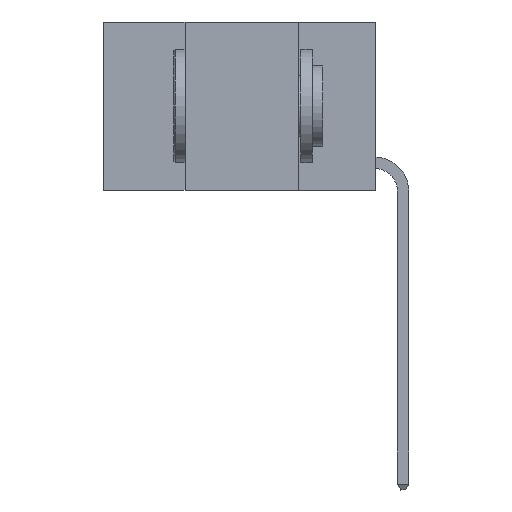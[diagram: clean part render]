
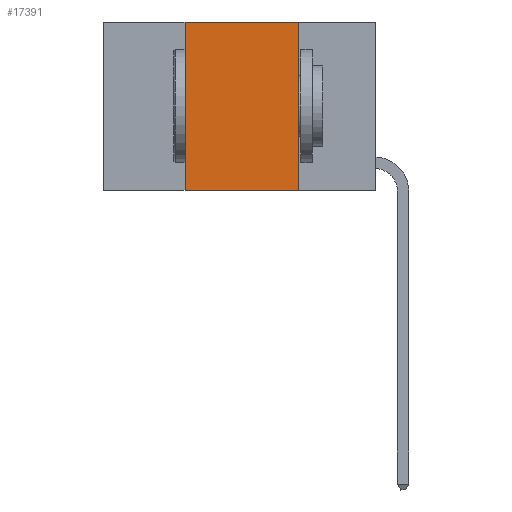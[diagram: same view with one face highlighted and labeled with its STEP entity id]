
A CAD part, left-side view. The second image highlights one B-rep face of the part: STEP entity #17391.
In plain terms, the highlighted planar face has unit normal (-1, 0, 0).
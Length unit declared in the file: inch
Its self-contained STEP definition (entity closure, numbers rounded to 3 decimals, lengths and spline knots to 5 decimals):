
#11 = CARTESIAN_POINT ( 'NONE',  ( 0., 0.17, 0. ) ) ;
#609 = EDGE_CURVE ( 'NONE', #15413, #7336, #24005, .T. ) ;
#3359 = VECTOR ( 'NONE', #26243, 39.37008 ) ;
#3717 = EDGE_CURVE ( 'NONE', #7336, #6108, #17285, .T. ) ;
#4016 = DIRECTION ( 'NONE',  ( 0., -1., 0. ) ) ;
#5914 = DIRECTION ( 'NONE',  ( 0., 0., 1. ) ) ;
#6108 = VERTEX_POINT ( 'NONE', #11 ) ;
#7336 = VERTEX_POINT ( 'NONE', #24976 ) ;
#7759 = CARTESIAN_POINT ( 'NONE',  ( 0., 0.6, 0. ) ) ;
#8882 = EDGE_LOOP ( 'NONE', ( #19151, #16259, #11368, #23279 ) ) ;
#9271 = CARTESIAN_POINT ( 'NONE',  ( 0., 0.42, -0.37 ) ) ;
#9733 = LINE ( 'NONE', #20394, #16869 ) ;
#10546 = VECTOR ( 'NONE', #5914, 39.37008 ) ;
#11368 = ORIENTED_EDGE ( 'NONE', *, *, #609, .F. ) ;
#11575 = PLANE ( 'NONE',  #26871 ) ;
#12954 = LINE ( 'NONE', #23762, #3359 ) ;
#15413 = VERTEX_POINT ( 'NONE', #9271 ) ;
#16259 = ORIENTED_EDGE ( 'NONE', *, *, #3717, .F. ) ;
#16667 = DIRECTION ( 'NONE',  ( 0., 0., -1. ) ) ;
#16869 = VECTOR ( 'NONE', #18506, 39.37008 ) ;
#17285 = LINE ( 'NONE', #21812, #26152 ) ;
#17391 = ADVANCED_FACE ( 'NONE', ( #27766 ), #11575, .F. ) ;
#17561 = VERTEX_POINT ( 'NONE', #19858 ) ;
#18299 = DIRECTION ( 'NONE',  ( 1., 0., 0. ) ) ;
#18506 = DIRECTION ( 'NONE',  ( 0., -1., 0. ) ) ;
#19151 = ORIENTED_EDGE ( 'NONE', *, *, #28224, .F. ) ;
#19858 = CARTESIAN_POINT ( 'NONE',  ( 0., 0.17, -0.37 ) ) ;
#20394 = CARTESIAN_POINT ( 'NONE',  ( 0., 0.6, -0.37 ) ) ;
#21812 = CARTESIAN_POINT ( 'NONE',  ( 0., 0.6, 0. ) ) ;
#21951 = CARTESIAN_POINT ( 'NONE',  ( 0., 0.42, 0. ) ) ;
#23279 = ORIENTED_EDGE ( 'NONE', *, *, #28581, .T. ) ;
#23762 = CARTESIAN_POINT ( 'NONE',  ( 0., 0.17, 0. ) ) ;
#24005 = LINE ( 'NONE', #21951, #10546 ) ;
#24976 = CARTESIAN_POINT ( 'NONE',  ( 0., 0.42, 0. ) ) ;
#26152 = VECTOR ( 'NONE', #4016, 39.37008 ) ;
#26243 = DIRECTION ( 'NONE',  ( 0., 0., -1. ) ) ;
#26871 = AXIS2_PLACEMENT_3D ( 'NONE', #7759, #18299, #16667 ) ;
#27766 = FACE_OUTER_BOUND ( 'NONE', #8882, .T. ) ;
#28224 = EDGE_CURVE ( 'NONE', #6108, #17561, #12954, .T. ) ;
#28581 = EDGE_CURVE ( 'NONE', #15413, #17561, #9733, .T. ) ;
